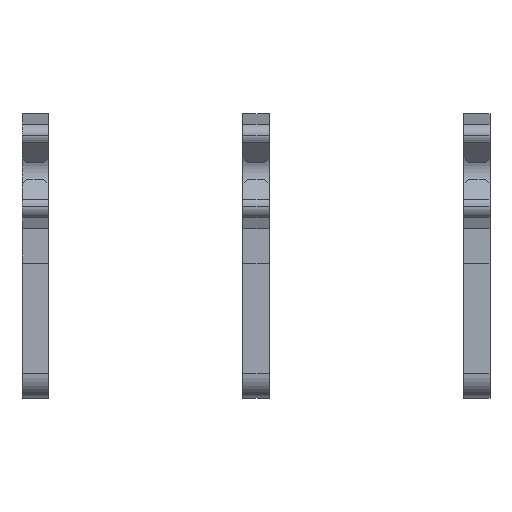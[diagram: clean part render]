
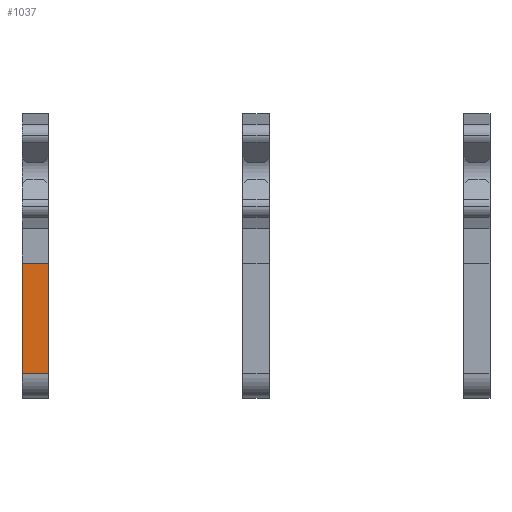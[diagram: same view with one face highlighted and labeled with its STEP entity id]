
A CAD part, top view. The second image highlights one B-rep face of the part: STEP entity #1037.
In plain terms, the highlighted planar face has unit normal (0, 0, 1).
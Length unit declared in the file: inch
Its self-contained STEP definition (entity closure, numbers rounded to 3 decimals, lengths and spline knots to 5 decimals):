
#10 = CARTESIAN_POINT ( 'NONE',  ( 0.0118, -0.183, -0.058 ) ) ;
#39 = ORIENTED_EDGE ( 'NONE', *, *, #1168, .F. ) ;
#59 = DIRECTION ( 'NONE',  ( 0., -1., 0. ) ) ;
#61 = CARTESIAN_POINT ( 'NONE',  ( -0.0118, -0.183, -0.058 ) ) ;
#65 = VECTOR ( 'NONE', #499, 39.37008 ) ;
#82 = VECTOR ( 'NONE', #1002, 39.37008 ) ;
#85 = DIRECTION ( 'NONE',  ( 0., -1., 0. ) ) ;
#95 = LINE ( 'NONE', #10, #65 ) ;
#98 = LINE ( 'NONE', #339, #82 ) ;
#108 = VECTOR ( 'NONE', #59, 39.37008 ) ;
#167 = VERTEX_POINT ( 'NONE', #1085 ) ;
#209 = FACE_OUTER_BOUND ( 'NONE', #569, .T. ) ;
#216 = EDGE_CURVE ( 'NONE', #167, #1224, #367, .T. ) ;
#289 = CARTESIAN_POINT ( 'NONE',  ( 0.0118, -0.183, -0.058 ) ) ;
#339 = CARTESIAN_POINT ( 'NONE',  ( 0.0118, -0.083, -0.058 ) ) ;
#367 = LINE ( 'NONE', #61, #108 ) ;
#377 = PLANE ( 'NONE',  #939 ) ;
#387 = DIRECTION ( 'NONE',  ( -1., 0., 0. ) ) ;
#462 = EDGE_CURVE ( 'NONE', #986, #703, #636, .T. ) ;
#468 = VECTOR ( 'NONE', #85, 39.37008 ) ;
#499 = DIRECTION ( 'NONE',  ( -1., 0., 0. ) ) ;
#535 = CARTESIAN_POINT ( 'NONE',  ( 0.0118, -0.183, -0.058 ) ) ;
#569 = EDGE_LOOP ( 'NONE', ( #1019, #39, #1146, #712 ) ) ;
#636 = LINE ( 'NONE', #1035, #468 ) ;
#703 = VERTEX_POINT ( 'NONE', #535 ) ;
#712 = ORIENTED_EDGE ( 'NONE', *, *, #744, .T. ) ;
#744 = EDGE_CURVE ( 'NONE', #986, #167, #98, .T. ) ;
#754 = CARTESIAN_POINT ( 'NONE',  ( 0.0118, -0.083, -0.058 ) ) ;
#939 = AXIS2_PLACEMENT_3D ( 'NONE', #289, #964, #387 ) ;
#964 = DIRECTION ( 'NONE',  ( 0., 0., -1. ) ) ;
#986 = VERTEX_POINT ( 'NONE', #754 ) ;
#1002 = DIRECTION ( 'NONE',  ( -1., 0., 0. ) ) ;
#1019 = ORIENTED_EDGE ( 'NONE', *, *, #216, .T. ) ;
#1035 = CARTESIAN_POINT ( 'NONE',  ( 0.0118, -0.183, -0.058 ) ) ;
#1037 = ADVANCED_FACE ( 'NONE', ( #209 ), #377, .F. ) ;
#1085 = CARTESIAN_POINT ( 'NONE',  ( -0.0118, -0.083, -0.058 ) ) ;
#1091 = CARTESIAN_POINT ( 'NONE',  ( -0.0118, -0.183, -0.058 ) ) ;
#1146 = ORIENTED_EDGE ( 'NONE', *, *, #462, .F. ) ;
#1168 = EDGE_CURVE ( 'NONE', #703, #1224, #95, .T. ) ;
#1224 = VERTEX_POINT ( 'NONE', #1091 ) ;
